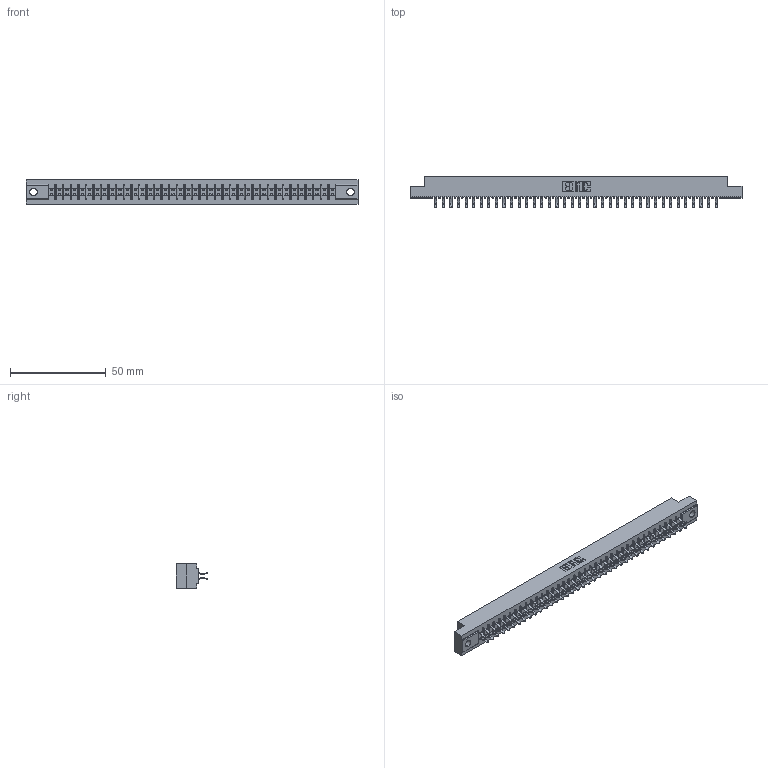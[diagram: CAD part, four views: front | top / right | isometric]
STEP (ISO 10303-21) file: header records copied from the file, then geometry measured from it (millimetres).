
FILE_DESCRIPTION (( 'STEP AP203' ), '1' );
FILE_NAME ('315-076-556-204.STEP', '2019-09-10T22:37:00', ( '' ), ( '' ), 'SwSTEP 2.0', 'SolidWorks 2016', '' );
FILE_SCHEMA (( 'CONFIG_CONTROL_DESIGN' ));
Length unit declared in the file: inch
Products named in the file (3): 305-290-001_556; 305 Part_.156 Dia; 315-076-556-204
Assembly tree (77 placements, depth 2):
  315-076-556-204
    305 Part_.156 Dia
    305-290-001_556  x76
Bounding box: 173.58 x 16.64 x 12.7 mm (x, y, z)
Volume: 17969.6 mm3; surface area: 22628.2 mm2
Topology: 77 solids, 77 shells, 4386 faces, 12626 edges, 8212 vertices
Faces by surface type: plane 2438, cylinder 1796, sphere 152
Entity records: 42271 total; most frequent: CARTESIAN_POINT 7002, ORIENTED_EDGE 6948, DIRECTION 6772, EDGE_CURVE 3474, LINE 2808, VECTOR 2808, VERTEX_POINT 2212, AXIS2_PLACEMENT_3D 1982
